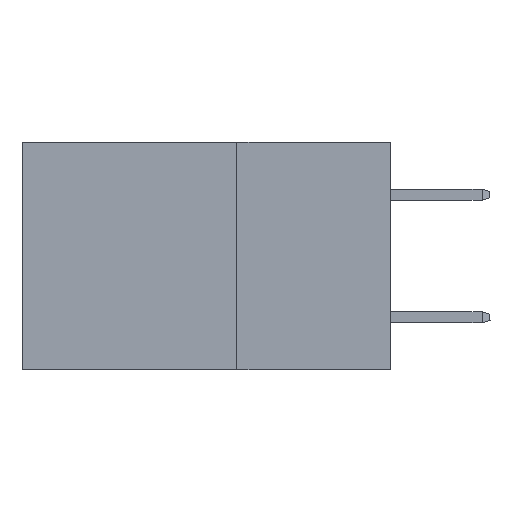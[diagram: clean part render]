
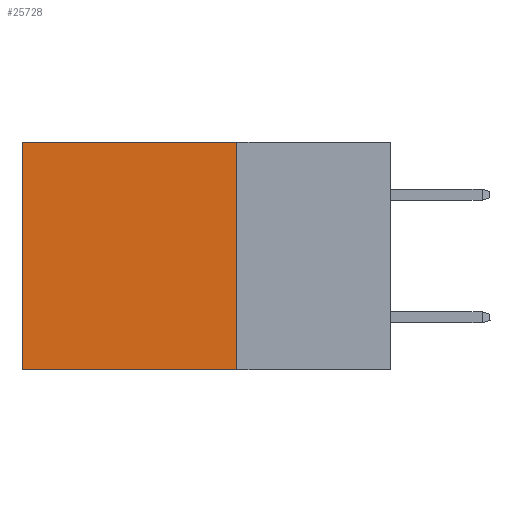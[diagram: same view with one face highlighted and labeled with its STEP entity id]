
A CAD part, left-side view. The second image highlights one B-rep face of the part: STEP entity #25728.
In plain terms, the highlighted planar face has unit normal (-1, 0, 0).
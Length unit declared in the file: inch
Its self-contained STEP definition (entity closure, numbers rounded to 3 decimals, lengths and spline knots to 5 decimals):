
#94 = DIRECTION ( 'NONE',  ( 0., 0., -1. ) ) ;
#930 = DIRECTION ( 'NONE',  ( 0., 1., 0. ) ) ;
#3214 = VECTOR ( 'NONE', #15805, 39.37008 ) ;
#3267 = VECTOR ( 'NONE', #21965, 39.37008 ) ;
#4029 = CARTESIAN_POINT ( 'NONE',  ( 0.2875, 0.25, -0.37 ) ) ;
#4457 = ORIENTED_EDGE ( 'NONE', *, *, #19351, .F. ) ;
#4880 = CARTESIAN_POINT ( 'NONE',  ( 0.2875, 0.25, -0.37 ) ) ;
#5415 = AXIS2_PLACEMENT_3D ( 'NONE', #14925, #22538, #27047 ) ;
#7301 = ORIENTED_EDGE ( 'NONE', *, *, #25140, .T. ) ;
#7601 = VECTOR ( 'NONE', #94, 39.37008 ) ;
#9040 = LINE ( 'NONE', #4880, #3267 ) ;
#9577 = VERTEX_POINT ( 'NONE', #20617 ) ;
#9755 = LINE ( 'NONE', #20636, #3214 ) ;
#9958 = EDGE_CURVE ( 'NONE', #13731, #9577, #18734, .T. ) ;
#10874 = VERTEX_POINT ( 'NONE', #22918 ) ;
#13126 = ORIENTED_EDGE ( 'NONE', *, *, #9958, .T. ) ;
#13731 = VERTEX_POINT ( 'NONE', #23177 ) ;
#14789 = VERTEX_POINT ( 'NONE', #4029 ) ;
#14925 = CARTESIAN_POINT ( 'NONE',  ( 0.2875, 0.25, 0. ) ) ;
#15805 = DIRECTION ( 'NONE',  ( 0., 0., -1. ) ) ;
#18734 = LINE ( 'NONE', #27682, #23313 ) ;
#19350 = EDGE_LOOP ( 'NONE', ( #7301, #21972, #4457, #13126 ) ) ;
#19351 = EDGE_CURVE ( 'NONE', #13731, #14789, #9755, .T. ) ;
#19668 = PLANE ( 'NONE',  #5415 ) ;
#19960 = CARTESIAN_POINT ( 'NONE',  ( 0.2875, 0.6, 0. ) ) ;
#20617 = CARTESIAN_POINT ( 'NONE',  ( 0.2875, 0.6, 0. ) ) ;
#20636 = CARTESIAN_POINT ( 'NONE',  ( 0.2875, 0.25, 0. ) ) ;
#21739 = LINE ( 'NONE', #19960, #7601 ) ;
#21965 = DIRECTION ( 'NONE',  ( 0., 1., 0. ) ) ;
#21972 = ORIENTED_EDGE ( 'NONE', *, *, #28118, .F. ) ;
#22538 = DIRECTION ( 'NONE',  ( 1., 0., 0. ) ) ;
#22918 = CARTESIAN_POINT ( 'NONE',  ( 0.2875, 0.6, -0.37 ) ) ;
#23177 = CARTESIAN_POINT ( 'NONE',  ( 0.2875, 0.25, 0. ) ) ;
#23313 = VECTOR ( 'NONE', #930, 39.37008 ) ;
#25140 = EDGE_CURVE ( 'NONE', #9577, #10874, #21739, .T. ) ;
#25728 = ADVANCED_FACE ( 'NONE', ( #30527 ), #19668, .F. ) ;
#27047 = DIRECTION ( 'NONE',  ( 0., 0., -1. ) ) ;
#27682 = CARTESIAN_POINT ( 'NONE',  ( 0.2875, 0.25, 0. ) ) ;
#28118 = EDGE_CURVE ( 'NONE', #14789, #10874, #9040, .T. ) ;
#30527 = FACE_OUTER_BOUND ( 'NONE', #19350, .T. ) ;
